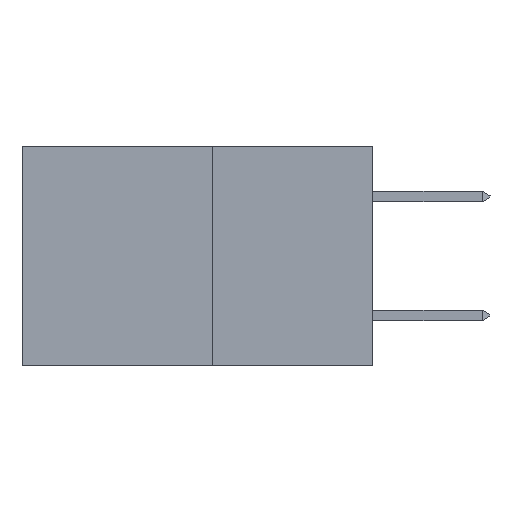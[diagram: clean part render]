
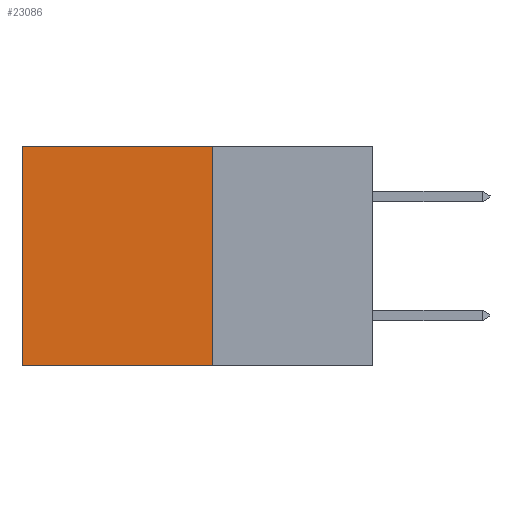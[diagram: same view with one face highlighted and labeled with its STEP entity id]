
A CAD part, left-side view. The second image highlights one B-rep face of the part: STEP entity #23086.
In plain terms, the highlighted planar face has unit normal (-1, 0, 0).
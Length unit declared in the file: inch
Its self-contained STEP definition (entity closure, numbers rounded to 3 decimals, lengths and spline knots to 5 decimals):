
#54 = ORIENTED_EDGE ( 'NONE', *, *, #24820, .F. ) ;
#351 = CARTESIAN_POINT ( 'NONE',  ( 0.277, 0.27, -0.37 ) ) ;
#783 = DIRECTION ( 'NONE',  ( 0., 0., -1. ) ) ;
#1810 = CARTESIAN_POINT ( 'NONE',  ( 0.277, 0.59, -0.37 ) ) ;
#2737 = LINE ( 'NONE', #19356, #23357 ) ;
#2751 = VERTEX_POINT ( 'NONE', #5118 ) ;
#5118 = CARTESIAN_POINT ( 'NONE',  ( 0.277, 0.27, 0. ) ) ;
#7173 = VECTOR ( 'NONE', #23222, 39.37008 ) ;
#7179 = VERTEX_POINT ( 'NONE', #351 ) ;
#7740 = ORIENTED_EDGE ( 'NONE', *, *, #18290, .F. ) ;
#7936 = CARTESIAN_POINT ( 'NONE',  ( 0.277, 0.27, -0.37 ) ) ;
#8079 = ORIENTED_EDGE ( 'NONE', *, *, #21805, .T. ) ;
#8655 = EDGE_CURVE ( 'NONE', #17171, #24343, #2737, .T. ) ;
#8739 = LINE ( 'NONE', #7936, #24414 ) ;
#9758 = DIRECTION ( 'NONE',  ( 0., 1., 0. ) ) ;
#9798 = PLANE ( 'NONE',  #14211 ) ;
#10008 = DIRECTION ( 'NONE',  ( 0., 0., -1. ) ) ;
#10960 = CARTESIAN_POINT ( 'NONE',  ( 0.277, 0.27, -0.37 ) ) ;
#11726 = CARTESIAN_POINT ( 'NONE',  ( 0.277, 0.59, 0. ) ) ;
#11944 = DIRECTION ( 'NONE',  ( 0., 0., -1. ) ) ;
#14211 = AXIS2_PLACEMENT_3D ( 'NONE', #22150, #24195, #11944 ) ;
#14499 = EDGE_LOOP ( 'NONE', ( #25263, #7740, #54, #8079 ) ) ;
#17171 = VERTEX_POINT ( 'NONE', #11726 ) ;
#18104 = LINE ( 'NONE', #10960, #7173 ) ;
#18290 = EDGE_CURVE ( 'NONE', #7179, #24343, #18104, .T. ) ;
#19356 = CARTESIAN_POINT ( 'NONE',  ( 0.277, 0.59, -0.37 ) ) ;
#21753 = VECTOR ( 'NONE', #9758, 39.37008 ) ;
#21805 = EDGE_CURVE ( 'NONE', #2751, #17171, #25227, .T. ) ;
#22150 = CARTESIAN_POINT ( 'NONE',  ( 0.277, 0.27, -0.37 ) ) ;
#23086 = ADVANCED_FACE ( 'NONE', ( #25150 ), #9798, .F. ) ;
#23222 = DIRECTION ( 'NONE',  ( 0., 1., 0. ) ) ;
#23357 = VECTOR ( 'NONE', #783, 39.37008 ) ;
#24078 = CARTESIAN_POINT ( 'NONE',  ( 0.277, 0.27, 0. ) ) ;
#24195 = DIRECTION ( 'NONE',  ( 1., 0., 0. ) ) ;
#24343 = VERTEX_POINT ( 'NONE', #1810 ) ;
#24414 = VECTOR ( 'NONE', #10008, 39.37008 ) ;
#24820 = EDGE_CURVE ( 'NONE', #2751, #7179, #8739, .T. ) ;
#25150 = FACE_OUTER_BOUND ( 'NONE', #14499, .T. ) ;
#25227 = LINE ( 'NONE', #24078, #21753 ) ;
#25263 = ORIENTED_EDGE ( 'NONE', *, *, #8655, .T. ) ;
